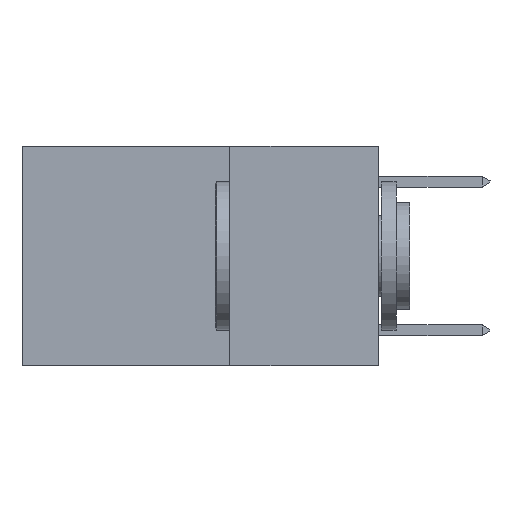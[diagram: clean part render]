
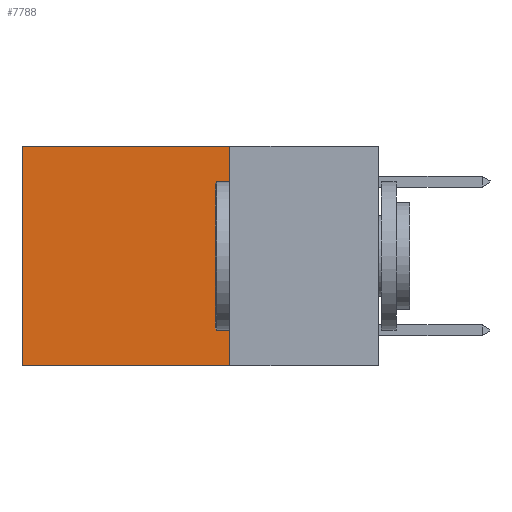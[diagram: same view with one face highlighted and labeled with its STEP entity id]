
A CAD part, left-side view. The second image highlights one B-rep face of the part: STEP entity #7788.
In plain terms, the highlighted planar face has unit normal (-1, 0, 0).
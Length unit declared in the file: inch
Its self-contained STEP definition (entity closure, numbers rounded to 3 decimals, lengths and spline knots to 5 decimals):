
#343 = CARTESIAN_POINT ( 'NONE',  ( 0.2625, 0.25, 0. ) ) ;
#997 = EDGE_CURVE ( 'NONE', #1949, #6991, #1189, .T. ) ;
#1189 = LINE ( 'NONE', #5073, #7042 ) ;
#1420 = DIRECTION ( 'NONE',  ( 0., 0., -1. ) ) ;
#1506 = ORIENTED_EDGE ( 'NONE', *, *, #997, .T. ) ;
#1949 = VERTEX_POINT ( 'NONE', #4753 ) ;
#2293 = VECTOR ( 'NONE', #9683, 39.37008 ) ;
#2930 = PLANE ( 'NONE',  #5982 ) ;
#3155 = CARTESIAN_POINT ( 'NONE',  ( 0.2625, 0.6, -0.37 ) ) ;
#3541 = FACE_OUTER_BOUND ( 'NONE', #3915, .T. ) ;
#3571 = CARTESIAN_POINT ( 'NONE',  ( 0.2625, 0.25, -0.37 ) ) ;
#3886 = DIRECTION ( 'NONE',  ( 0., 0., -1. ) ) ;
#3915 = EDGE_LOOP ( 'NONE', ( #1506, #6274, #6380, #5615 ) ) ;
#3974 = CARTESIAN_POINT ( 'NONE',  ( 0.2625, 0.25, 0. ) ) ;
#4238 = EDGE_CURVE ( 'NONE', #7126, #1949, #7890, .T. ) ;
#4319 = LINE ( 'NONE', #3571, #2293 ) ;
#4753 = CARTESIAN_POINT ( 'NONE',  ( 0.2625, 0.6, 0. ) ) ;
#4811 = CARTESIAN_POINT ( 'NONE',  ( 0.2625, 0.25, 0. ) ) ;
#5073 = CARTESIAN_POINT ( 'NONE',  ( 0.2625, 0.6, 0. ) ) ;
#5223 = VECTOR ( 'NONE', #8609, 39.37008 ) ;
#5615 = ORIENTED_EDGE ( 'NONE', *, *, #4238, .T. ) ;
#5685 = VERTEX_POINT ( 'NONE', #6828 ) ;
#5781 = VECTOR ( 'NONE', #6481, 39.37008 ) ;
#5911 = LINE ( 'NONE', #3974, #5223 ) ;
#5976 = DIRECTION ( 'NONE',  ( 1., 0., 0. ) ) ;
#5982 = AXIS2_PLACEMENT_3D ( 'NONE', #6720, #5976, #1420 ) ;
#6274 = ORIENTED_EDGE ( 'NONE', *, *, #6634, .F. ) ;
#6380 = ORIENTED_EDGE ( 'NONE', *, *, #7974, .F. ) ;
#6481 = DIRECTION ( 'NONE',  ( 0., 1., 0. ) ) ;
#6634 = EDGE_CURVE ( 'NONE', #5685, #6991, #4319, .T. ) ;
#6720 = CARTESIAN_POINT ( 'NONE',  ( 0.2625, 0.25, 0. ) ) ;
#6828 = CARTESIAN_POINT ( 'NONE',  ( 0.2625, 0.25, -0.37 ) ) ;
#6991 = VERTEX_POINT ( 'NONE', #3155 ) ;
#7042 = VECTOR ( 'NONE', #3886, 39.37008 ) ;
#7126 = VERTEX_POINT ( 'NONE', #4811 ) ;
#7788 = ADVANCED_FACE ( 'NONE', ( #3541 ), #2930, .F. ) ;
#7890 = LINE ( 'NONE', #343, #5781 ) ;
#7974 = EDGE_CURVE ( 'NONE', #7126, #5685, #5911, .T. ) ;
#8609 = DIRECTION ( 'NONE',  ( 0., 0., -1. ) ) ;
#9683 = DIRECTION ( 'NONE',  ( 0., 1., 0. ) ) ;
